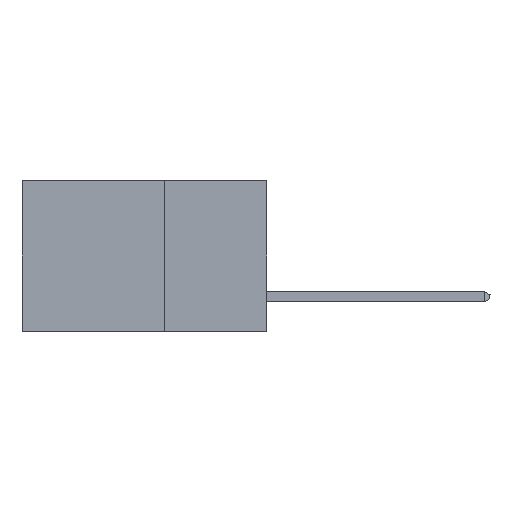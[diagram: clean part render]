
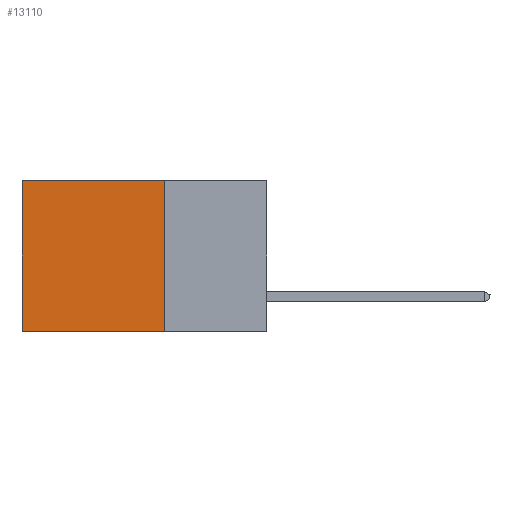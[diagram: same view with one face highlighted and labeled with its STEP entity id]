
A CAD part, left-side view. The second image highlights one B-rep face of the part: STEP entity #13110.
In plain terms, the highlighted planar face has unit normal (-1, 0, 0).
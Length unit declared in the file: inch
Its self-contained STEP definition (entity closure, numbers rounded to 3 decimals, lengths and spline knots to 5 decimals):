
#2310 = EDGE_LOOP ( 'NONE', ( #5798, #7700, #10192, #19080 ) ) ;
#2673 = CARTESIAN_POINT ( 'NONE',  ( 0.2875, 0.25, -0.37 ) ) ;
#3719 = EDGE_CURVE ( 'NONE', #24702, #5737, #10221, .T. ) ;
#4796 = DIRECTION ( 'NONE',  ( 0., 1., 0. ) ) ;
#4974 = CARTESIAN_POINT ( 'NONE',  ( 0.2875, 0.25, 0. ) ) ;
#5737 = VERTEX_POINT ( 'NONE', #14348 ) ;
#5798 = ORIENTED_EDGE ( 'NONE', *, *, #3719, .T. ) ;
#5806 = LINE ( 'NONE', #20410, #20905 ) ;
#7305 = EDGE_CURVE ( 'NONE', #22328, #29535, #31390, .T. ) ;
#7700 = ORIENTED_EDGE ( 'NONE', *, *, #10516, .F. ) ;
#7788 = AXIS2_PLACEMENT_3D ( 'NONE', #19743, #22284, #24860 ) ;
#9323 = CARTESIAN_POINT ( 'NONE',  ( 0.2875, 0.25, -0.37 ) ) ;
#10192 = ORIENTED_EDGE ( 'NONE', *, *, #7305, .F. ) ;
#10221 = LINE ( 'NONE', #17257, #15286 ) ;
#10516 = EDGE_CURVE ( 'NONE', #29535, #5737, #31911, .T. ) ;
#11596 = FACE_OUTER_BOUND ( 'NONE', #2310, .T. ) ;
#13110 = ADVANCED_FACE ( 'NONE', ( #11596 ), #17178, .F. ) ;
#14348 = CARTESIAN_POINT ( 'NONE',  ( 0.2875, 0.6, -0.37 ) ) ;
#14996 = DIRECTION ( 'NONE',  ( 0., 1., 0. ) ) ;
#15162 = DIRECTION ( 'NONE',  ( 0., 0., -1. ) ) ;
#15203 = VECTOR ( 'NONE', #15162, 39.37008 ) ;
#15286 = VECTOR ( 'NONE', #24816, 39.37008 ) ;
#17178 = PLANE ( 'NONE',  #7788 ) ;
#17257 = CARTESIAN_POINT ( 'NONE',  ( 0.2875, 0.6, 0. ) ) ;
#17326 = VECTOR ( 'NONE', #14996, 39.37008 ) ;
#18715 = CARTESIAN_POINT ( 'NONE',  ( 0.2875, 0.6, 0. ) ) ;
#19080 = ORIENTED_EDGE ( 'NONE', *, *, #25420, .T. ) ;
#19743 = CARTESIAN_POINT ( 'NONE',  ( 0.2875, 0.25, 0. ) ) ;
#20410 = CARTESIAN_POINT ( 'NONE',  ( 0.2875, 0.25, 0. ) ) ;
#20905 = VECTOR ( 'NONE', #4796, 39.37008 ) ;
#22284 = DIRECTION ( 'NONE',  ( 1., 0., 0. ) ) ;
#22328 = VERTEX_POINT ( 'NONE', #30612 ) ;
#24702 = VERTEX_POINT ( 'NONE', #18715 ) ;
#24816 = DIRECTION ( 'NONE',  ( 0., 0., -1. ) ) ;
#24860 = DIRECTION ( 'NONE',  ( 0., 0., -1. ) ) ;
#25420 = EDGE_CURVE ( 'NONE', #22328, #24702, #5806, .T. ) ;
#29535 = VERTEX_POINT ( 'NONE', #9323 ) ;
#30612 = CARTESIAN_POINT ( 'NONE',  ( 0.2875, 0.25, 0. ) ) ;
#31390 = LINE ( 'NONE', #4974, #15203 ) ;
#31911 = LINE ( 'NONE', #2673, #17326 ) ;
